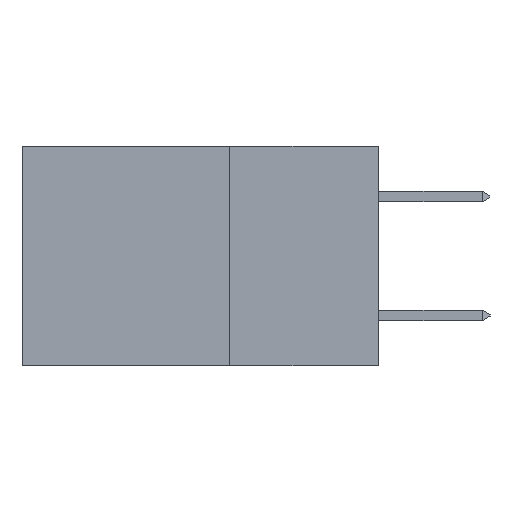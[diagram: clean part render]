
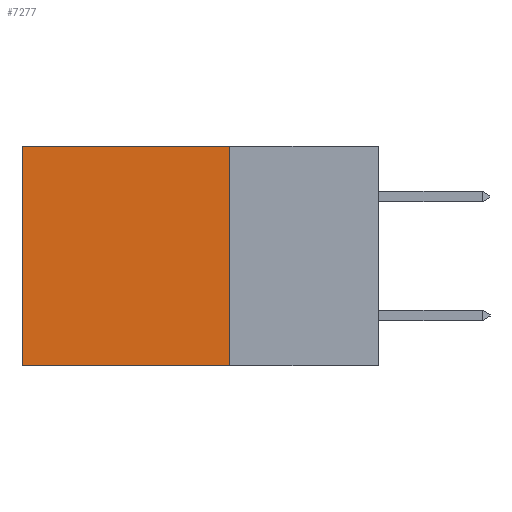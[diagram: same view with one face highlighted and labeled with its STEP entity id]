
A CAD part, left-side view. The second image highlights one B-rep face of the part: STEP entity #7277.
In plain terms, the highlighted planar face has unit normal (-1, 0, 0).
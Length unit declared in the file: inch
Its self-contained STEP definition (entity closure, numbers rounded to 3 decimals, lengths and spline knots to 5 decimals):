
#386 = VERTEX_POINT ( 'NONE', #1227 ) ;
#727 = CARTESIAN_POINT ( 'NONE',  ( 0.2615, 0.25, -0.37 ) ) ;
#1133 = DIRECTION ( 'NONE',  ( 0., 0., -1. ) ) ;
#1227 = CARTESIAN_POINT ( 'NONE',  ( 0.2615, 0.6, -0.37 ) ) ;
#2447 = VERTEX_POINT ( 'NONE', #18521 ) ;
#2789 = VECTOR ( 'NONE', #8845, 39.37008 ) ;
#3124 = EDGE_CURVE ( 'NONE', #13792, #386, #3770, .T. ) ;
#3325 = ORIENTED_EDGE ( 'NONE', *, *, #4711, .F. ) ;
#3770 = LINE ( 'NONE', #20370, #2789 ) ;
#4323 = CARTESIAN_POINT ( 'NONE',  ( 0.2615, 0.25, -0.37 ) ) ;
#4711 = EDGE_CURVE ( 'NONE', #2447, #12394, #7002, .T. ) ;
#6349 = DIRECTION ( 'NONE',  ( 0., 1., 0. ) ) ;
#7002 = LINE ( 'NONE', #727, #11169 ) ;
#7277 = ADVANCED_FACE ( 'NONE', ( #12754 ), #12458, .F. ) ;
#7511 = EDGE_LOOP ( 'NONE', ( #7606, #9061, #3325, #12793 ) ) ;
#7606 = ORIENTED_EDGE ( 'NONE', *, *, #3124, .T. ) ;
#7651 = LINE ( 'NONE', #10740, #11326 ) ;
#8845 = DIRECTION ( 'NONE',  ( 0., 0., -1. ) ) ;
#9061 = ORIENTED_EDGE ( 'NONE', *, *, #15470, .F. ) ;
#9636 = LINE ( 'NONE', #19044, #12360 ) ;
#10740 = CARTESIAN_POINT ( 'NONE',  ( 0.2615, 0.25, 0. ) ) ;
#11169 = VECTOR ( 'NONE', #1133, 39.37008 ) ;
#11326 = VECTOR ( 'NONE', #18670, 39.37008 ) ;
#12360 = VECTOR ( 'NONE', #6349, 39.37008 ) ;
#12394 = VERTEX_POINT ( 'NONE', #4323 ) ;
#12399 = DIRECTION ( 'NONE',  ( 0., 0., -1. ) ) ;
#12431 = DIRECTION ( 'NONE',  ( 1., 0., 0. ) ) ;
#12453 = CARTESIAN_POINT ( 'NONE',  ( 0.2615, 0.25, -0.37 ) ) ;
#12458 = PLANE ( 'NONE',  #19103 ) ;
#12754 = FACE_OUTER_BOUND ( 'NONE', #7511, .T. ) ;
#12793 = ORIENTED_EDGE ( 'NONE', *, *, #16017, .T. ) ;
#13792 = VERTEX_POINT ( 'NONE', #20243 ) ;
#15470 = EDGE_CURVE ( 'NONE', #12394, #386, #9636, .T. ) ;
#16017 = EDGE_CURVE ( 'NONE', #2447, #13792, #7651, .T. ) ;
#18521 = CARTESIAN_POINT ( 'NONE',  ( 0.2615, 0.25, 0. ) ) ;
#18670 = DIRECTION ( 'NONE',  ( 0., 1., 0. ) ) ;
#19044 = CARTESIAN_POINT ( 'NONE',  ( 0.2615, 0.25, -0.37 ) ) ;
#19103 = AXIS2_PLACEMENT_3D ( 'NONE', #12453, #12431, #12399 ) ;
#20243 = CARTESIAN_POINT ( 'NONE',  ( 0.2615, 0.6, 0. ) ) ;
#20370 = CARTESIAN_POINT ( 'NONE',  ( 0.2615, 0.6, -0.37 ) ) ;
